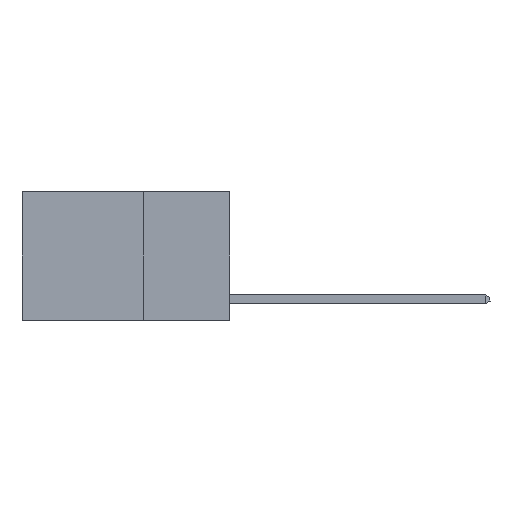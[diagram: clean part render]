
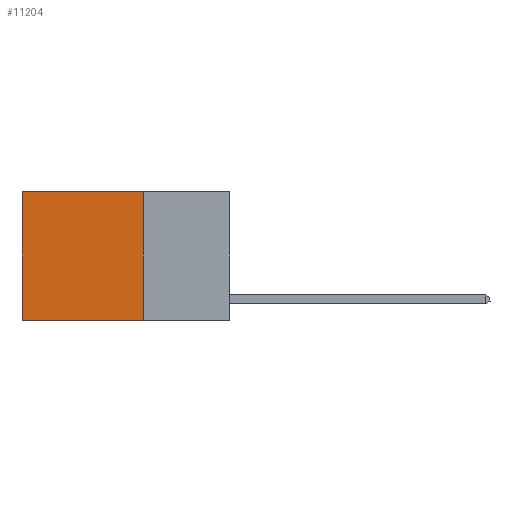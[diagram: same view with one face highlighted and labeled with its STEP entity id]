
A CAD part, left-side view. The second image highlights one B-rep face of the part: STEP entity #11204.
In plain terms, the highlighted planar face has unit normal (-1, 0, 0).
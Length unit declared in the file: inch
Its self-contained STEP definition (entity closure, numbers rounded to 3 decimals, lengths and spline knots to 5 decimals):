
#1044 = ORIENTED_EDGE ( 'NONE', *, *, #16669, .F. ) ;
#2397 = VERTEX_POINT ( 'NONE', #7566 ) ;
#2701 = EDGE_CURVE ( 'NONE', #15059, #4226, #10466, .T. ) ;
#2827 = ORIENTED_EDGE ( 'NONE', *, *, #12784, .F. ) ;
#2901 = CARTESIAN_POINT ( 'NONE',  ( 0.2625, 0.6, -0.37 ) ) ;
#3878 = VECTOR ( 'NONE', #9015, 39.37008 ) ;
#4149 = VECTOR ( 'NONE', #11289, 39.37008 ) ;
#4226 = VERTEX_POINT ( 'NONE', #2901 ) ;
#4747 = DIRECTION ( 'NONE',  ( 0., 0., -1. ) ) ;
#4798 = CARTESIAN_POINT ( 'NONE',  ( 0.2625, 0.6, 0. ) ) ;
#6533 = CARTESIAN_POINT ( 'NONE',  ( 0.2625, 0.25, 0. ) ) ;
#7347 = CARTESIAN_POINT ( 'NONE',  ( 0.2625, 0.25, -0.37 ) ) ;
#7566 = CARTESIAN_POINT ( 'NONE',  ( 0.2625, 0.25, 0. ) ) ;
#7688 = CARTESIAN_POINT ( 'NONE',  ( 0.2625, 0.25, 0. ) ) ;
#7695 = AXIS2_PLACEMENT_3D ( 'NONE', #13014, #7701, #16938 ) ;
#7701 = DIRECTION ( 'NONE',  ( 1., 0., 0. ) ) ;
#8464 = VECTOR ( 'NONE', #15823, 39.37008 ) ;
#9015 = DIRECTION ( 'NONE',  ( 0., 0., -1. ) ) ;
#9170 = VERTEX_POINT ( 'NONE', #14189 ) ;
#9344 = EDGE_CURVE ( 'NONE', #2397, #15059, #11550, .T. ) ;
#9416 = ORIENTED_EDGE ( 'NONE', *, *, #2701, .T. ) ;
#9593 = EDGE_LOOP ( 'NONE', ( #9416, #2827, #1044, #14238 ) ) ;
#10466 = LINE ( 'NONE', #4798, #17047 ) ;
#10845 = LINE ( 'NONE', #7347, #4149 ) ;
#10997 = LINE ( 'NONE', #7688, #3878 ) ;
#11204 = ADVANCED_FACE ( 'NONE', ( #15102 ), #14365, .F. ) ;
#11289 = DIRECTION ( 'NONE',  ( 0., 1., 0. ) ) ;
#11550 = LINE ( 'NONE', #6533, #8464 ) ;
#12784 = EDGE_CURVE ( 'NONE', #9170, #4226, #10845, .T. ) ;
#13014 = CARTESIAN_POINT ( 'NONE',  ( 0.2625, 0.25, 0. ) ) ;
#14189 = CARTESIAN_POINT ( 'NONE',  ( 0.2625, 0.25, -0.37 ) ) ;
#14238 = ORIENTED_EDGE ( 'NONE', *, *, #9344, .T. ) ;
#14365 = PLANE ( 'NONE',  #7695 ) ;
#15059 = VERTEX_POINT ( 'NONE', #17304 ) ;
#15102 = FACE_OUTER_BOUND ( 'NONE', #9593, .T. ) ;
#15823 = DIRECTION ( 'NONE',  ( 0., 1., 0. ) ) ;
#16669 = EDGE_CURVE ( 'NONE', #2397, #9170, #10997, .T. ) ;
#16938 = DIRECTION ( 'NONE',  ( 0., 0., -1. ) ) ;
#17047 = VECTOR ( 'NONE', #4747, 39.37008 ) ;
#17304 = CARTESIAN_POINT ( 'NONE',  ( 0.2625, 0.6, 0. ) ) ;
